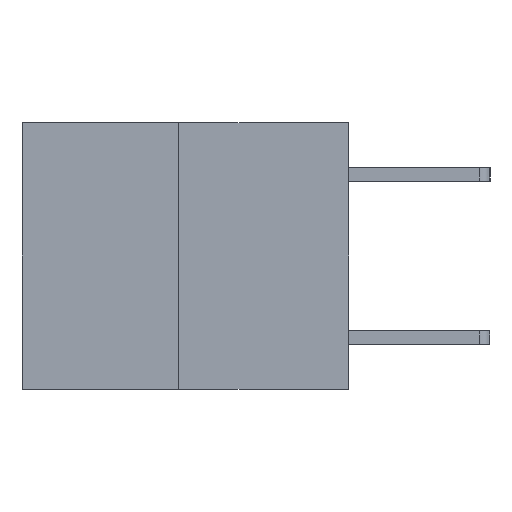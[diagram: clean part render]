
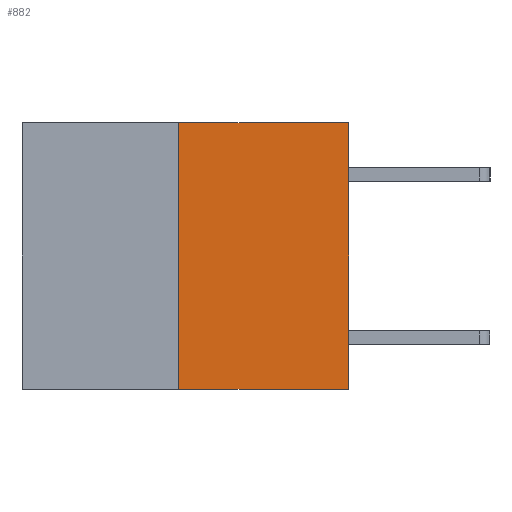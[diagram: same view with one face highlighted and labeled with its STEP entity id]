
A CAD part, left-side view. The second image highlights one B-rep face of the part: STEP entity #882.
In plain terms, the highlighted planar face has unit normal (-1, 0, 0).
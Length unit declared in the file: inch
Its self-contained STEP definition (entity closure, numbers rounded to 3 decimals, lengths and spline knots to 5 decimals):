
#6 = DIRECTION ( 'NONE',  ( 0., -1., 0. ) ) ;
#388 = AXIS2_PLACEMENT_3D ( 'NONE', #8144, #10859, #9998 ) ;
#882 = ADVANCED_FACE ( 'NONE', ( #6867 ), #1832, .F. ) ;
#1215 = CARTESIAN_POINT ( 'NONE',  ( 0., 0., -0.49 ) ) ;
#1361 = VERTEX_POINT ( 'NONE', #9586 ) ;
#1364 = DIRECTION ( 'NONE',  ( 0., 0., 1. ) ) ;
#1446 = CARTESIAN_POINT ( 'NONE',  ( 0., 0.312, -0.49 ) ) ;
#1556 = CARTESIAN_POINT ( 'NONE',  ( 0., 0.6, 0. ) ) ;
#1832 = PLANE ( 'NONE',  #388 ) ;
#2251 = ORIENTED_EDGE ( 'NONE', *, *, #10602, .F. ) ;
#3092 = LINE ( 'NONE', #6543, #11029 ) ;
#3287 = DIRECTION ( 'NONE',  ( 0., -1., 0. ) ) ;
#4302 = ORIENTED_EDGE ( 'NONE', *, *, #7652, .T. ) ;
#4495 = CARTESIAN_POINT ( 'NONE',  ( 0., 0.6, -0.49 ) ) ;
#5203 = VECTOR ( 'NONE', #3287, 39.37008 ) ;
#5676 = LINE ( 'NONE', #4495, #7200 ) ;
#5821 = VERTEX_POINT ( 'NONE', #1446 ) ;
#5829 = CARTESIAN_POINT ( 'NONE',  ( 0., 0., 0. ) ) ;
#6359 = VECTOR ( 'NONE', #1364, 39.37008 ) ;
#6543 = CARTESIAN_POINT ( 'NONE',  ( 0., 0.312, -0.49 ) ) ;
#6806 = VERTEX_POINT ( 'NONE', #11009 ) ;
#6867 = FACE_OUTER_BOUND ( 'NONE', #8158, .T. ) ;
#7200 = VECTOR ( 'NONE', #6, 39.37008 ) ;
#7396 = VERTEX_POINT ( 'NONE', #1215 ) ;
#7652 = EDGE_CURVE ( 'NONE', #5821, #7396, #5676, .T. ) ;
#7740 = EDGE_CURVE ( 'NONE', #7396, #1361, #11192, .T. ) ;
#8144 = CARTESIAN_POINT ( 'NONE',  ( 0., 0.6, 0. ) ) ;
#8158 = EDGE_LOOP ( 'NONE', ( #2251, #4302, #11526, #11105 ) ) ;
#8532 = EDGE_CURVE ( 'NONE', #6806, #1361, #11712, .T. ) ;
#9338 = DIRECTION ( 'NONE',  ( 0., 0., 1. ) ) ;
#9586 = CARTESIAN_POINT ( 'NONE',  ( 0., 0., 0. ) ) ;
#9998 = DIRECTION ( 'NONE',  ( 0., 0., -1. ) ) ;
#10602 = EDGE_CURVE ( 'NONE', #5821, #6806, #3092, .T. ) ;
#10859 = DIRECTION ( 'NONE',  ( 1., 0., 0. ) ) ;
#11009 = CARTESIAN_POINT ( 'NONE',  ( 0., 0.312, 0. ) ) ;
#11029 = VECTOR ( 'NONE', #9338, 39.37008 ) ;
#11105 = ORIENTED_EDGE ( 'NONE', *, *, #8532, .F. ) ;
#11192 = LINE ( 'NONE', #5829, #6359 ) ;
#11526 = ORIENTED_EDGE ( 'NONE', *, *, #7740, .T. ) ;
#11712 = LINE ( 'NONE', #1556, #5203 ) ;
